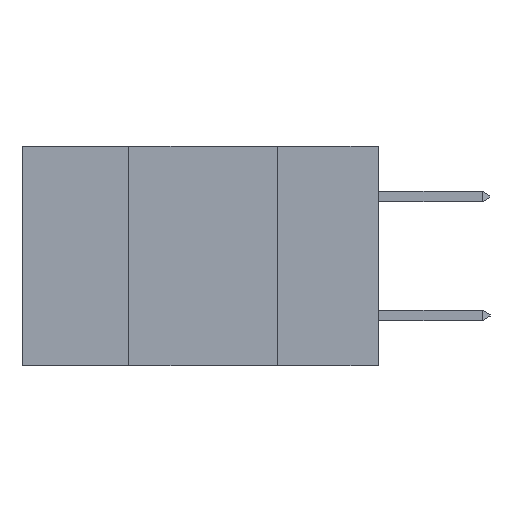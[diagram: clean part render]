
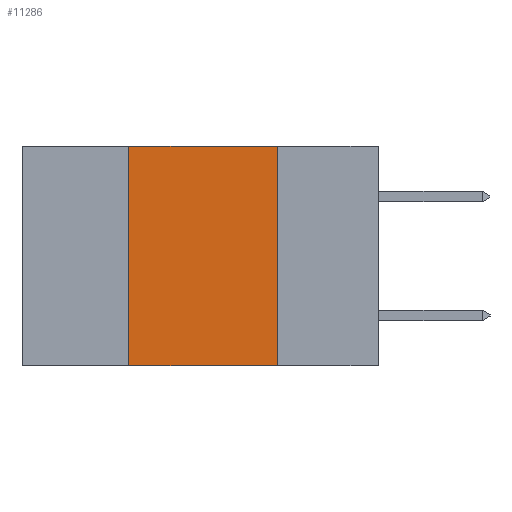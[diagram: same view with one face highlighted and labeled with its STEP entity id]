
A CAD part, left-side view. The second image highlights one B-rep face of the part: STEP entity #11286.
In plain terms, the highlighted planar face has unit normal (-1, 0, 0).
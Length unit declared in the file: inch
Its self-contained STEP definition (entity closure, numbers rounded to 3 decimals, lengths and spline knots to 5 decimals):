
#2351 = CARTESIAN_POINT ( 'NONE',  ( 0., 0.17, -0.37 ) ) ;
#2437 = EDGE_LOOP ( 'NONE', ( #10933, #16674, #20771, #5974 ) ) ;
#4332 = DIRECTION ( 'NONE',  ( 0., -1., 0. ) ) ;
#4394 = EDGE_CURVE ( 'NONE', #12381, #24664, #11545, .T. ) ;
#4667 = DIRECTION ( 'NONE',  ( 0., 0., -1. ) ) ;
#5809 = DIRECTION ( 'NONE',  ( 0., -1., 0. ) ) ;
#5974 = ORIENTED_EDGE ( 'NONE', *, *, #4394, .T. ) ;
#9878 = VECTOR ( 'NONE', #21305, 39.37008 ) ;
#10933 = ORIENTED_EDGE ( 'NONE', *, *, #23044, .F. ) ;
#11286 = ADVANCED_FACE ( 'NONE', ( #22491 ), #14763, .F. ) ;
#11459 = CARTESIAN_POINT ( 'NONE',  ( 0., 0.17, 0. ) ) ;
#11545 = LINE ( 'NONE', #15891, #23423 ) ;
#12381 = VERTEX_POINT ( 'NONE', #14267 ) ;
#13216 = LINE ( 'NONE', #18395, #23179 ) ;
#13883 = LINE ( 'NONE', #19802, #18548 ) ;
#13886 = AXIS2_PLACEMENT_3D ( 'NONE', #16665, #16756, #4667 ) ;
#14267 = CARTESIAN_POINT ( 'NONE',  ( 0., 0.42, -0.37 ) ) ;
#14763 = PLANE ( 'NONE',  #13886 ) ;
#15275 = LINE ( 'NONE', #17299, #9878 ) ;
#15891 = CARTESIAN_POINT ( 'NONE',  ( 0., 0.6, -0.37 ) ) ;
#16045 = CARTESIAN_POINT ( 'NONE',  ( 0., 0.42, 0. ) ) ;
#16665 = CARTESIAN_POINT ( 'NONE',  ( 0., 0.6, 0. ) ) ;
#16674 = ORIENTED_EDGE ( 'NONE', *, *, #16993, .F. ) ;
#16756 = DIRECTION ( 'NONE',  ( 1., 0., 0. ) ) ;
#16993 = EDGE_CURVE ( 'NONE', #18569, #17350, #13216, .T. ) ;
#17299 = CARTESIAN_POINT ( 'NONE',  ( 0., 0.42, -0.37 ) ) ;
#17350 = VERTEX_POINT ( 'NONE', #11459 ) ;
#18395 = CARTESIAN_POINT ( 'NONE',  ( 0., 0.6, 0. ) ) ;
#18548 = VECTOR ( 'NONE', #21811, 39.37008 ) ;
#18569 = VERTEX_POINT ( 'NONE', #16045 ) ;
#19802 = CARTESIAN_POINT ( 'NONE',  ( 0., 0.17, -0.37 ) ) ;
#20732 = EDGE_CURVE ( 'NONE', #12381, #18569, #15275, .T. ) ;
#20771 = ORIENTED_EDGE ( 'NONE', *, *, #20732, .F. ) ;
#21305 = DIRECTION ( 'NONE',  ( 0., 0., 1. ) ) ;
#21811 = DIRECTION ( 'NONE',  ( 0., 0., -1. ) ) ;
#22491 = FACE_OUTER_BOUND ( 'NONE', #2437, .T. ) ;
#23044 = EDGE_CURVE ( 'NONE', #17350, #24664, #13883, .T. ) ;
#23179 = VECTOR ( 'NONE', #4332, 39.37008 ) ;
#23423 = VECTOR ( 'NONE', #5809, 39.37008 ) ;
#24664 = VERTEX_POINT ( 'NONE', #2351 ) ;
